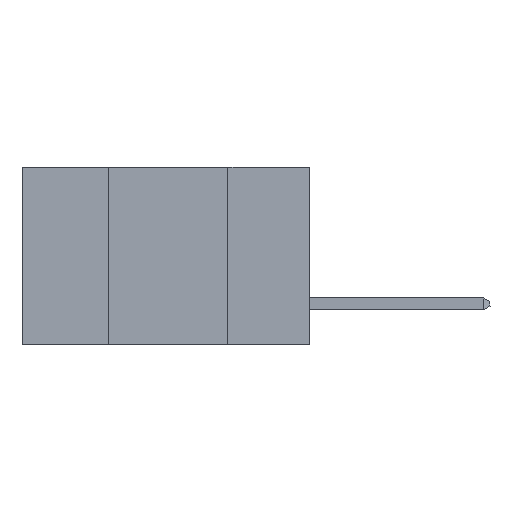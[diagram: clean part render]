
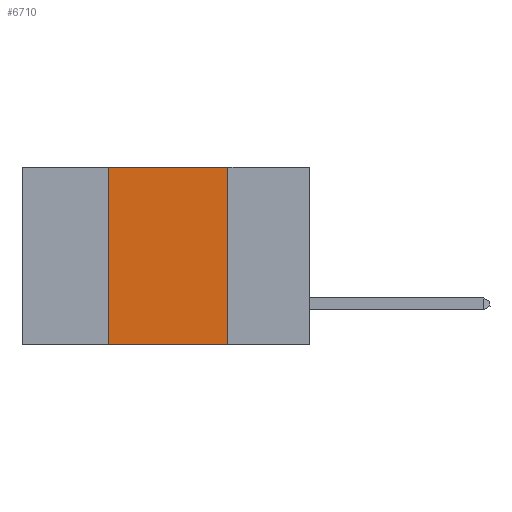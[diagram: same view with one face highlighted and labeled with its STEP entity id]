
A CAD part, left-side view. The second image highlights one B-rep face of the part: STEP entity #6710.
In plain terms, the highlighted planar face has unit normal (-1, 0, 0).
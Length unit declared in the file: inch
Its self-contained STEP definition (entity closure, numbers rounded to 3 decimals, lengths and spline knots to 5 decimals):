
#63 = CARTESIAN_POINT ( 'NONE',  ( 0., 0.6, 0. ) ) ;
#846 = CARTESIAN_POINT ( 'NONE',  ( 0., 0.42, 0. ) ) ;
#861 = CARTESIAN_POINT ( 'NONE',  ( 0., 0.42, -0.37 ) ) ;
#1452 = LINE ( 'NONE', #846, #11711 ) ;
#1918 = VECTOR ( 'NONE', #13438, 39.37008 ) ;
#2237 = DIRECTION ( 'NONE',  ( 1., 0., 0. ) ) ;
#4511 = VERTEX_POINT ( 'NONE', #861 ) ;
#5514 = CARTESIAN_POINT ( 'NONE',  ( 0., 0.42, 0. ) ) ;
#5890 = VERTEX_POINT ( 'NONE', #5514 ) ;
#6124 = CARTESIAN_POINT ( 'NONE',  ( 0., 0.17, -0.37 ) ) ;
#6393 = CARTESIAN_POINT ( 'NONE',  ( 0., 0.17, 0. ) ) ;
#6710 = ADVANCED_FACE ( 'NONE', ( #14948 ), #12417, .F. ) ;
#6834 = EDGE_CURVE ( 'NONE', #4511, #18084, #11817, .T. ) ;
#10847 = ORIENTED_EDGE ( 'NONE', *, *, #6834, .T. ) ;
#11690 = LINE ( 'NONE', #12036, #18268 ) ;
#11711 = VECTOR ( 'NONE', #23051, 39.37008 ) ;
#11758 = ORIENTED_EDGE ( 'NONE', *, *, #19063, .F. ) ;
#11817 = LINE ( 'NONE', #16785, #12441 ) ;
#12036 = CARTESIAN_POINT ( 'NONE',  ( 0., 0.6, 0. ) ) ;
#12151 = LINE ( 'NONE', #17470, #1918 ) ;
#12174 = EDGE_LOOP ( 'NONE', ( #16360, #14920, #11758, #10847 ) ) ;
#12417 = PLANE ( 'NONE',  #23662 ) ;
#12441 = VECTOR ( 'NONE', #18826, 39.37008 ) ;
#13438 = DIRECTION ( 'NONE',  ( 0., 0., -1. ) ) ;
#14920 = ORIENTED_EDGE ( 'NONE', *, *, #19490, .F. ) ;
#14948 = FACE_OUTER_BOUND ( 'NONE', #12174, .T. ) ;
#16360 = ORIENTED_EDGE ( 'NONE', *, *, #23013, .F. ) ;
#16432 = DIRECTION ( 'NONE',  ( 0., 0., -1. ) ) ;
#16785 = CARTESIAN_POINT ( 'NONE',  ( 0., 0.6, -0.37 ) ) ;
#17470 = CARTESIAN_POINT ( 'NONE',  ( 0., 0.17, 0. ) ) ;
#18084 = VERTEX_POINT ( 'NONE', #6124 ) ;
#18268 = VECTOR ( 'NONE', #25926, 39.37008 ) ;
#18826 = DIRECTION ( 'NONE',  ( 0., -1., 0. ) ) ;
#19063 = EDGE_CURVE ( 'NONE', #4511, #5890, #1452, .T. ) ;
#19490 = EDGE_CURVE ( 'NONE', #5890, #23377, #11690, .T. ) ;
#23013 = EDGE_CURVE ( 'NONE', #23377, #18084, #12151, .T. ) ;
#23051 = DIRECTION ( 'NONE',  ( 0., 0., 1. ) ) ;
#23377 = VERTEX_POINT ( 'NONE', #6393 ) ;
#23662 = AXIS2_PLACEMENT_3D ( 'NONE', #63, #2237, #16432 ) ;
#25926 = DIRECTION ( 'NONE',  ( 0., -1., 0. ) ) ;
